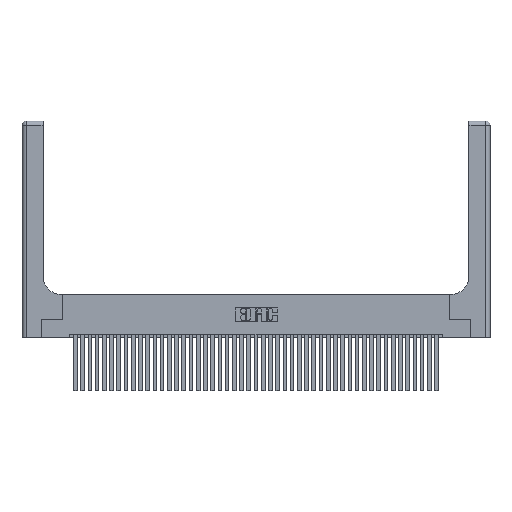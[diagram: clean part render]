
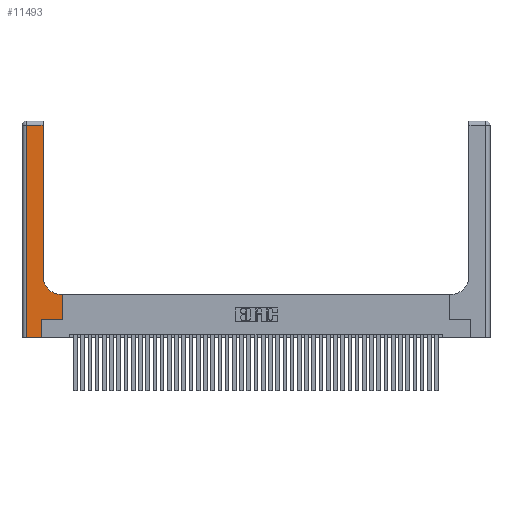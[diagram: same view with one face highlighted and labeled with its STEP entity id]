
A CAD part, top view. The second image highlights one B-rep face of the part: STEP entity #11493.
In plain terms, the highlighted planar face has unit normal (0, 0, 1).
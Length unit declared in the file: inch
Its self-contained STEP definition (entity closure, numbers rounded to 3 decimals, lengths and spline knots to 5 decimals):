
#944 = DIRECTION ( 'NONE',  ( 0., 0., -1. ) ) ;
#1180 = CARTESIAN_POINT ( 'NONE',  ( 0.5585, 0.25, 0.37 ) ) ;
#1182 = EDGE_CURVE ( 'NONE', #8069, #2061, #11603, .T. ) ;
#1568 = CIRCLE ( 'NONE', #11539, 0.25 ) ;
#1728 = CARTESIAN_POINT ( 'NONE',  ( 0.5415, 0.6, 0.37 ) ) ;
#1795 = DIRECTION ( 'NONE',  ( 1., 0., 0. ) ) ;
#2061 = VERTEX_POINT ( 'NONE', #1728 ) ;
#2293 = EDGE_CURVE ( 'NONE', #20532, #29350, #5528, .T. ) ;
#2583 = VECTOR ( 'NONE', #3730, 39.37008 ) ;
#2732 = EDGE_CURVE ( 'NONE', #33990, #20532, #36285, .T. ) ;
#2746 = ORIENTED_EDGE ( 'NONE', *, *, #1182, .T. ) ;
#2837 = DIRECTION ( 'NONE',  ( 0., 1., 0. ) ) ;
#3730 = DIRECTION ( 'NONE',  ( -1., 0., 0. ) ) ;
#4084 = VECTOR ( 'NONE', #13632, 39.37008 ) ;
#4983 = VECTOR ( 'NONE', #2837, 39.37008 ) ;
#5528 = LINE ( 'NONE', #18063, #23593 ) ;
#7250 = VERTEX_POINT ( 'NONE', #24651 ) ;
#7506 = VECTOR ( 'NONE', #30702, 39.37008 ) ;
#8069 = VERTEX_POINT ( 'NONE', #35612 ) ;
#8588 = VECTOR ( 'NONE', #15772, 39.37008 ) ;
#8928 = ORIENTED_EDGE ( 'NONE', *, *, #26355, .T. ) ;
#10170 = LINE ( 'NONE', #30267, #7506 ) ;
#10301 = CARTESIAN_POINT ( 'NONE',  ( 0.269, 0.25, 0.37 ) ) ;
#11493 = ADVANCED_FACE ( 'NONE', ( #25568 ), #11748, .F. ) ;
#11539 = AXIS2_PLACEMENT_3D ( 'NONE', #19269, #11868, #1795 ) ;
#11603 = LINE ( 'NONE', #20513, #2583 ) ;
#11748 = PLANE ( 'NONE',  #35399 ) ;
#11868 = DIRECTION ( 'NONE',  ( 0., 0., -1. ) ) ;
#12743 = ORIENTED_EDGE ( 'NONE', *, *, #36096, .T. ) ;
#13632 = DIRECTION ( 'NONE',  ( 1., 0., 0. ) ) ;
#13751 = CARTESIAN_POINT ( 'NONE',  ( 0.06, 3., 0.37 ) ) ;
#14074 = EDGE_CURVE ( 'NONE', #2061, #31368, #1568, .T. ) ;
#14249 = VECTOR ( 'NONE', #35144, 39.37008 ) ;
#15510 = LINE ( 'NONE', #16661, #8588 ) ;
#15772 = DIRECTION ( 'NONE',  ( -1., 0., 0. ) ) ;
#16346 = LINE ( 'NONE', #37237, #4084 ) ;
#16661 = CARTESIAN_POINT ( 'NONE',  ( 0., 2.94, 0.37 ) ) ;
#16936 = ORIENTED_EDGE ( 'NONE', *, *, #41841, .T. ) ;
#17465 = DIRECTION ( 'NONE',  ( 0., -1., 0. ) ) ;
#18063 = CARTESIAN_POINT ( 'NONE',  ( 0.269, 0.25, 0.37 ) ) ;
#18482 = EDGE_CURVE ( 'NONE', #7250, #33990, #16346, .T. ) ;
#18872 = VECTOR ( 'NONE', #17465, 39.37008 ) ;
#19103 = EDGE_LOOP ( 'NONE', ( #36428, #12743, #16936, #30354, #40696, #22841, #8928, #2746, #32485 ) ) ;
#19269 = CARTESIAN_POINT ( 'NONE',  ( 0.5415, 0.85, 0.37 ) ) ;
#19767 = VERTEX_POINT ( 'NONE', #23095 ) ;
#20513 = CARTESIAN_POINT ( 'NONE',  ( 0.2915, 0.6, 0.37 ) ) ;
#20532 = VERTEX_POINT ( 'NONE', #10301 ) ;
#21266 = CARTESIAN_POINT ( 'NONE',  ( 0., 3., 0.37 ) ) ;
#22841 = ORIENTED_EDGE ( 'NONE', *, *, #2293, .T. ) ;
#23095 = CARTESIAN_POINT ( 'NONE',  ( 0.06, 2.94, 0.37 ) ) ;
#23251 = VERTEX_POINT ( 'NONE', #39701 ) ;
#23593 = VECTOR ( 'NONE', #31870, 39.37008 ) ;
#24651 = CARTESIAN_POINT ( 'NONE',  ( 0.06, 0., 0.37 ) ) ;
#24820 = DIRECTION ( 'NONE',  ( -1., 0., 0. ) ) ;
#25568 = FACE_OUTER_BOUND ( 'NONE', #19103, .T. ) ;
#26355 = EDGE_CURVE ( 'NONE', #29350, #8069, #30181, .T. ) ;
#27771 = CARTESIAN_POINT ( 'NONE',  ( 0.269, 0., 0.37 ) ) ;
#29350 = VERTEX_POINT ( 'NONE', #38033 ) ;
#29873 = CARTESIAN_POINT ( 'NONE',  ( 0.269, 0., 0.37 ) ) ;
#30181 = LINE ( 'NONE', #1180, #14249 ) ;
#30267 = CARTESIAN_POINT ( 'NONE',  ( 0.2915, 3., 0.37 ) ) ;
#30354 = ORIENTED_EDGE ( 'NONE', *, *, #18482, .T. ) ;
#30702 = DIRECTION ( 'NONE',  ( 0., 1., 0. ) ) ;
#31368 = VERTEX_POINT ( 'NONE', #38666 ) ;
#31870 = DIRECTION ( 'NONE',  ( 1., 0., 0. ) ) ;
#32485 = ORIENTED_EDGE ( 'NONE', *, *, #14074, .T. ) ;
#33990 = VERTEX_POINT ( 'NONE', #27771 ) ;
#34264 = LINE ( 'NONE', #13751, #18872 ) ;
#35144 = DIRECTION ( 'NONE',  ( 0., 1., 0. ) ) ;
#35399 = AXIS2_PLACEMENT_3D ( 'NONE', #21266, #944, #24820 ) ;
#35612 = CARTESIAN_POINT ( 'NONE',  ( 0.5585, 0.6, 0.37 ) ) ;
#36096 = EDGE_CURVE ( 'NONE', #23251, #19767, #15510, .T. ) ;
#36285 = LINE ( 'NONE', #29873, #4983 ) ;
#36428 = ORIENTED_EDGE ( 'NONE', *, *, #38165, .T. ) ;
#37237 = CARTESIAN_POINT ( 'NONE',  ( 0., 0., 0.37 ) ) ;
#38033 = CARTESIAN_POINT ( 'NONE',  ( 0.5585, 0.25, 0.37 ) ) ;
#38165 = EDGE_CURVE ( 'NONE', #31368, #23251, #10170, .T. ) ;
#38666 = CARTESIAN_POINT ( 'NONE',  ( 0.2915, 0.85, 0.37 ) ) ;
#39701 = CARTESIAN_POINT ( 'NONE',  ( 0.2915, 2.94, 0.37 ) ) ;
#40696 = ORIENTED_EDGE ( 'NONE', *, *, #2732, .T. ) ;
#41841 = EDGE_CURVE ( 'NONE', #19767, #7250, #34264, .T. ) ;
